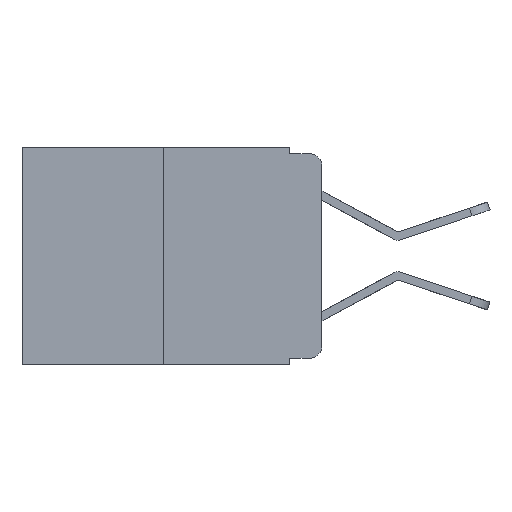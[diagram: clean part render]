
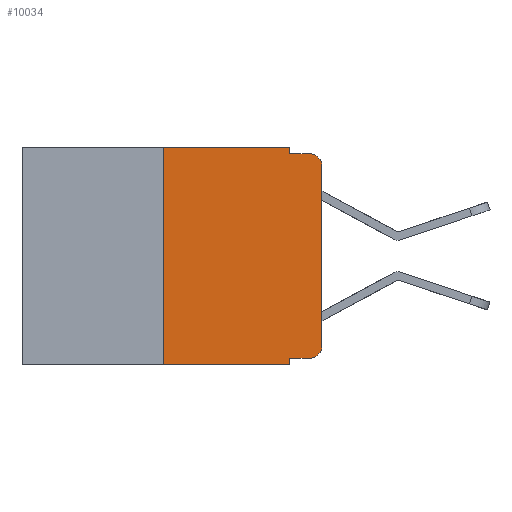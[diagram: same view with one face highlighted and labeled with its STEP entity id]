
A CAD part, left-side view. The second image highlights one B-rep face of the part: STEP entity #10034.
In plain terms, the highlighted planar face has unit normal (-1, 0, 0).
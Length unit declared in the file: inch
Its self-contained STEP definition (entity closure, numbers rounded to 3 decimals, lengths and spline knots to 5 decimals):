
#16 = VECTOR ( 'NONE', #24604, 39.37008 ) ;
#423 = DIRECTION ( 'NONE',  ( 0., -1., 0. ) ) ;
#462 = VERTEX_POINT ( 'NONE', #21755 ) ;
#619 = VERTEX_POINT ( 'NONE', #24511 ) ;
#993 = DIRECTION ( 'NONE',  ( -1., 0., 0. ) ) ;
#1052 = CARTESIAN_POINT ( 'NONE',  ( 0., 0.051, -0.01 ) ) ;
#1244 = CARTESIAN_POINT ( 'NONE',  ( 0., 0.473, -0.343 ) ) ;
#1505 = ORIENTED_EDGE ( 'NONE', *, *, #4338, .F. ) ;
#1865 = EDGE_CURVE ( 'NONE', #21967, #6454, #24448, .T. ) ;
#1914 = DIRECTION ( 'NONE',  ( 0., -1., 0. ) ) ;
#2524 = VERTEX_POINT ( 'NONE', #13442 ) ;
#2795 = AXIS2_PLACEMENT_3D ( 'NONE', #17169, #13502, #9466 ) ;
#2835 = DIRECTION ( 'NONE',  ( 0., 0., -1. ) ) ;
#2929 = DIRECTION ( 'NONE',  ( 0., 0., 1. ) ) ;
#3294 = EDGE_CURVE ( 'NONE', #619, #462, #7084, .T. ) ;
#3463 = CARTESIAN_POINT ( 'NONE',  ( 0., 0.051, 0. ) ) ;
#3621 = VERTEX_POINT ( 'NONE', #20384 ) ;
#4069 = VECTOR ( 'NONE', #2929, 39.37008 ) ;
#4129 = EDGE_CURVE ( 'NONE', #14287, #619, #5376, .T. ) ;
#4338 = EDGE_CURVE ( 'NONE', #2524, #12752, #22084, .T. ) ;
#4444 = LINE ( 'NONE', #1244, #14442 ) ;
#4761 = CARTESIAN_POINT ( 'NONE',  ( 0., 0.02, -0.313 ) ) ;
#5136 = DIRECTION ( 'NONE',  ( -1., 0., 0. ) ) ;
#5376 = LINE ( 'NONE', #24640, #7283 ) ;
#5672 = CARTESIAN_POINT ( 'NONE',  ( 0., 0., -0.03 ) ) ;
#6454 = VERTEX_POINT ( 'NONE', #21273 ) ;
#7052 = CARTESIAN_POINT ( 'NONE',  ( 0., 0., 0. ) ) ;
#7084 = LINE ( 'NONE', #12871, #16 ) ;
#7283 = VECTOR ( 'NONE', #13044, 39.37008 ) ;
#7559 = EDGE_CURVE ( 'NONE', #6454, #7744, #17998, .T. ) ;
#7744 = VERTEX_POINT ( 'NONE', #5672 ) ;
#8096 = VECTOR ( 'NONE', #2835, 39.37008 ) ;
#8462 = VERTEX_POINT ( 'NONE', #1052 ) ;
#8718 = LINE ( 'NONE', #19134, #23429 ) ;
#9067 = ORIENTED_EDGE ( 'NONE', *, *, #20817, .T. ) ;
#9466 = DIRECTION ( 'NONE',  ( 0., 0., -1. ) ) ;
#9836 = ORIENTED_EDGE ( 'NONE', *, *, #18360, .F. ) ;
#10034 = ADVANCED_FACE ( 'NONE', ( #22702 ), #21173, .F. ) ;
#11835 = EDGE_CURVE ( 'NONE', #462, #8462, #20683, .T. ) ;
#11994 = EDGE_CURVE ( 'NONE', #14287, #12752, #4444, .T. ) ;
#12208 = EDGE_LOOP ( 'NONE', ( #17831, #19571, #9836, #16196, #14411, #15595, #15030, #1505, #9067, #21416 ) ) ;
#12752 = VERTEX_POINT ( 'NONE', #17693 ) ;
#12871 = CARTESIAN_POINT ( 'NONE',  ( 0., 0.473, 0. ) ) ;
#13044 = DIRECTION ( 'NONE',  ( 0., 0., 1. ) ) ;
#13442 = CARTESIAN_POINT ( 'NONE',  ( 0., 0.051, -0.333 ) ) ;
#13502 = DIRECTION ( 'NONE',  ( 1., 0., 0. ) ) ;
#13658 = VECTOR ( 'NONE', #15415, 39.37008 ) ;
#13762 = CARTESIAN_POINT ( 'NONE',  ( 0., 0.02, -0.333 ) ) ;
#14287 = VERTEX_POINT ( 'NONE', #18311 ) ;
#14411 = ORIENTED_EDGE ( 'NONE', *, *, #3294, .F. ) ;
#14442 = VECTOR ( 'NONE', #423, 39.37008 ) ;
#15030 = ORIENTED_EDGE ( 'NONE', *, *, #11994, .T. ) ;
#15415 = DIRECTION ( 'NONE',  ( 0., 0., -1. ) ) ;
#15595 = ORIENTED_EDGE ( 'NONE', *, *, #4129, .F. ) ;
#16196 = ORIENTED_EDGE ( 'NONE', *, *, #11835, .F. ) ;
#16221 = EDGE_CURVE ( 'NONE', #7744, #3621, #20084, .T. ) ;
#16287 = VECTOR ( 'NONE', #18880, 39.37008 ) ;
#16306 = CARTESIAN_POINT ( 'NONE',  ( 0., 0.051, 0. ) ) ;
#16818 = AXIS2_PLACEMENT_3D ( 'NONE', #4761, #993, #18460 ) ;
#17169 = CARTESIAN_POINT ( 'NONE',  ( 0., 0.473, 0. ) ) ;
#17693 = CARTESIAN_POINT ( 'NONE',  ( 0., 0.051, -0.343 ) ) ;
#17831 = ORIENTED_EDGE ( 'NONE', *, *, #7559, .T. ) ;
#17998 = LINE ( 'NONE', #7052, #4069 ) ;
#18311 = CARTESIAN_POINT ( 'NONE',  ( 0., 0.25, -0.343 ) ) ;
#18360 = EDGE_CURVE ( 'NONE', #8462, #3621, #8718, .T. ) ;
#18460 = DIRECTION ( 'NONE',  ( 0., 0., -1. ) ) ;
#18471 = CARTESIAN_POINT ( 'NONE',  ( 0., 0.02, -0.03 ) ) ;
#18723 = DIRECTION ( 'NONE',  ( 0., 0., -1. ) ) ;
#18880 = DIRECTION ( 'NONE',  ( 0., -1., 0. ) ) ;
#19018 = LINE ( 'NONE', #22793, #16287 ) ;
#19134 = CARTESIAN_POINT ( 'NONE',  ( 0., 0.051, -0.01 ) ) ;
#19571 = ORIENTED_EDGE ( 'NONE', *, *, #16221, .T. ) ;
#20084 = CIRCLE ( 'NONE', #23332, 0.02 ) ;
#20384 = CARTESIAN_POINT ( 'NONE',  ( 0., 0.02, -0.01 ) ) ;
#20683 = LINE ( 'NONE', #3463, #13658 ) ;
#20817 = EDGE_CURVE ( 'NONE', #2524, #21967, #19018, .T. ) ;
#21173 = PLANE ( 'NONE',  #2795 ) ;
#21273 = CARTESIAN_POINT ( 'NONE',  ( 0., 0., -0.313 ) ) ;
#21416 = ORIENTED_EDGE ( 'NONE', *, *, #1865, .T. ) ;
#21755 = CARTESIAN_POINT ( 'NONE',  ( 0., 0.051, 0. ) ) ;
#21967 = VERTEX_POINT ( 'NONE', #13762 ) ;
#22084 = LINE ( 'NONE', #16306, #8096 ) ;
#22702 = FACE_OUTER_BOUND ( 'NONE', #12208, .T. ) ;
#22793 = CARTESIAN_POINT ( 'NONE',  ( 0., 0.051, -0.333 ) ) ;
#23332 = AXIS2_PLACEMENT_3D ( 'NONE', #18471, #5136, #18723 ) ;
#23429 = VECTOR ( 'NONE', #1914, 39.37008 ) ;
#24448 = CIRCLE ( 'NONE', #16818, 0.02 ) ;
#24511 = CARTESIAN_POINT ( 'NONE',  ( 0., 0.25, 0. ) ) ;
#24604 = DIRECTION ( 'NONE',  ( 0., -1., 0. ) ) ;
#24640 = CARTESIAN_POINT ( 'NONE',  ( 0., 0.25, 0. ) ) ;
